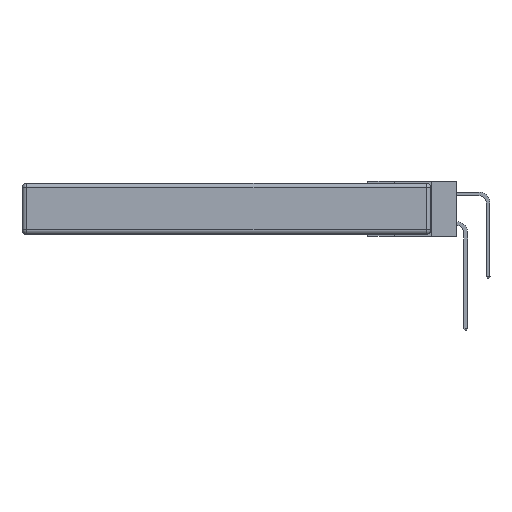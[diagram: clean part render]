
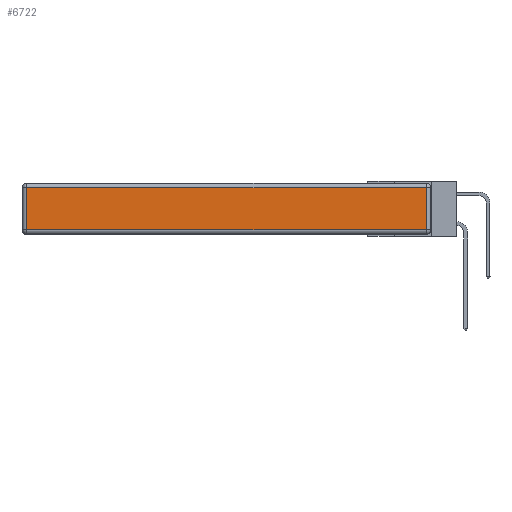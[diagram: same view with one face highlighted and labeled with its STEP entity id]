
A CAD part, left-side view. The second image highlights one B-rep face of the part: STEP entity #6722.
In plain terms, the highlighted planar face has unit normal (-1, 0, 0).
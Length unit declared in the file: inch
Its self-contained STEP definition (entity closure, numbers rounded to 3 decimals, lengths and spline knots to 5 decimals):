
#560 = CARTESIAN_POINT ( 'NONE',  ( 0., 0.03, -0.343 ) ) ;
#637 = DIRECTION ( 'NONE',  ( 0., 0., 1. ) ) ;
#1421 = DIRECTION ( 'NONE',  ( 0., 1., 0. ) ) ;
#1729 = AXIS2_PLACEMENT_3D ( 'NONE', #14210, #21695, #12586 ) ;
#2178 = LINE ( 'NONE', #23254, #18220 ) ;
#2246 = VECTOR ( 'NONE', #19239, 39.37008 ) ;
#2727 = CARTESIAN_POINT ( 'NONE',  ( 0., 2.72, -0.313 ) ) ;
#3109 = CARTESIAN_POINT ( 'NONE',  ( 0., 2.72, -0.343 ) ) ;
#3469 = EDGE_CURVE ( 'NONE', #7706, #15278, #21666, .T. ) ;
#3497 = EDGE_LOOP ( 'NONE', ( #20198, #20673, #12479, #21039 ) ) ;
#4249 = LINE ( 'NONE', #3109, #21446 ) ;
#5098 = LINE ( 'NONE', #10284, #2246 ) ;
#5252 = CARTESIAN_POINT ( 'NONE',  ( 0., 0.03, -0.313 ) ) ;
#6722 = ADVANCED_FACE ( 'NONE', ( #20660 ), #12503, .T. ) ;
#7706 = VERTEX_POINT ( 'NONE', #5252 ) ;
#8411 = VERTEX_POINT ( 'NONE', #9753 ) ;
#9582 = VERTEX_POINT ( 'NONE', #2727 ) ;
#9753 = CARTESIAN_POINT ( 'NONE',  ( 0., 2.72, -0.03 ) ) ;
#10284 = CARTESIAN_POINT ( 'NONE',  ( 0., 0., -0.313 ) ) ;
#11963 = EDGE_CURVE ( 'NONE', #8411, #9582, #4249, .T. ) ;
#12479 = ORIENTED_EDGE ( 'NONE', *, *, #20083, .T. ) ;
#12503 = PLANE ( 'NONE',  #1729 ) ;
#12586 = DIRECTION ( 'NONE',  ( 0., 0., 1. ) ) ;
#13098 = VECTOR ( 'NONE', #637, 39.37008 ) ;
#14210 = CARTESIAN_POINT ( 'NONE',  ( 0., 0., -0.343 ) ) ;
#14975 = CARTESIAN_POINT ( 'NONE',  ( 0., 0.03, -0.03 ) ) ;
#15278 = VERTEX_POINT ( 'NONE', #14975 ) ;
#18220 = VECTOR ( 'NONE', #1421, 39.37008 ) ;
#19239 = DIRECTION ( 'NONE',  ( 0., -1., 0. ) ) ;
#20083 = EDGE_CURVE ( 'NONE', #15278, #8411, #2178, .T. ) ;
#20198 = ORIENTED_EDGE ( 'NONE', *, *, #23285, .T. ) ;
#20660 = FACE_OUTER_BOUND ( 'NONE', #3497, .T. ) ;
#20673 = ORIENTED_EDGE ( 'NONE', *, *, #3469, .T. ) ;
#21039 = ORIENTED_EDGE ( 'NONE', *, *, #11963, .T. ) ;
#21327 = DIRECTION ( 'NONE',  ( 0., 0., -1. ) ) ;
#21446 = VECTOR ( 'NONE', #21327, 39.37008 ) ;
#21666 = LINE ( 'NONE', #560, #13098 ) ;
#21695 = DIRECTION ( 'NONE',  ( -1., 0., 0. ) ) ;
#23254 = CARTESIAN_POINT ( 'NONE',  ( 0., 2.75, -0.03 ) ) ;
#23285 = EDGE_CURVE ( 'NONE', #9582, #7706, #5098, .T. ) ;
